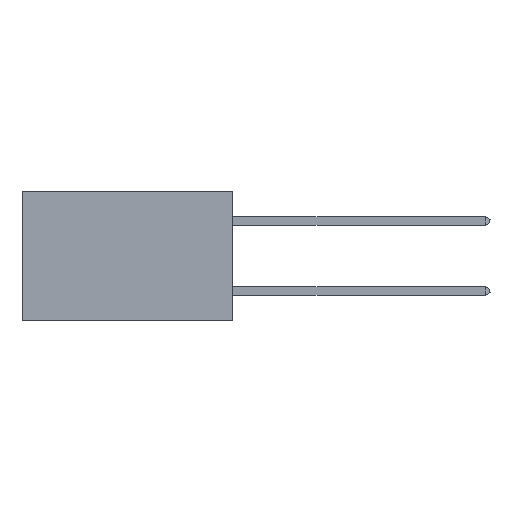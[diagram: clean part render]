
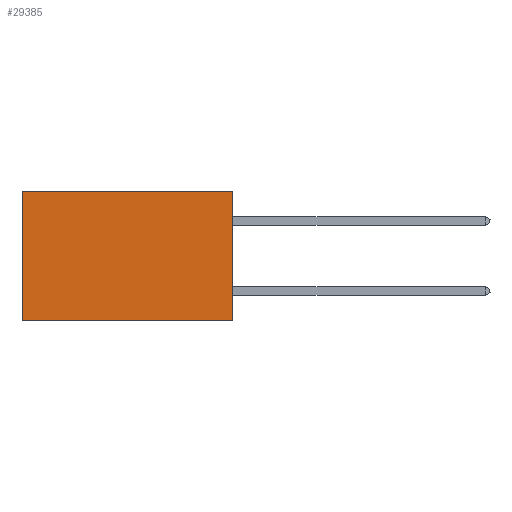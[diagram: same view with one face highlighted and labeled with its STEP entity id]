
A CAD part, left-side view. The second image highlights one B-rep face of the part: STEP entity #29385.
In plain terms, the highlighted planar face has unit normal (-1, 0, 0).
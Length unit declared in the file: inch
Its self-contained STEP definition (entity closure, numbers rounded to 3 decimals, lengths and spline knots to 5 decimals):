
#735 = VERTEX_POINT ( 'NONE', #17103 ) ;
#1496 = DIRECTION ( 'NONE',  ( 1., 0., 0. ) ) ;
#2989 = AXIS2_PLACEMENT_3D ( 'NONE', #29914, #1496, #18304 ) ;
#3746 = ORIENTED_EDGE ( 'NONE', *, *, #8281, .F. ) ;
#4450 = DIRECTION ( 'NONE',  ( 0., 0., -1. ) ) ;
#5558 = ORIENTED_EDGE ( 'NONE', *, *, #13737, .T. ) ;
#6247 = CARTESIAN_POINT ( 'NONE',  ( 0.2875, 0.6, -0.37 ) ) ;
#6467 = EDGE_LOOP ( 'NONE', ( #12537, #3746, #24023, #5558 ) ) ;
#7039 = VERTEX_POINT ( 'NONE', #28938 ) ;
#8281 = EDGE_CURVE ( 'NONE', #7039, #26730, #9430, .T. ) ;
#8569 = CARTESIAN_POINT ( 'NONE',  ( 0.2875, 0., 0. ) ) ;
#9321 = CARTESIAN_POINT ( 'NONE',  ( 0.2875, 0.6, 0. ) ) ;
#9430 = LINE ( 'NONE', #9608, #15730 ) ;
#9608 = CARTESIAN_POINT ( 'NONE',  ( 0.2875, 0., -0.37 ) ) ;
#11564 = LINE ( 'NONE', #14207, #23347 ) ;
#11989 = DIRECTION ( 'NONE',  ( 0., 1., 0. ) ) ;
#12326 = CARTESIAN_POINT ( 'NONE',  ( 0.2875, 0.6, 0. ) ) ;
#12537 = ORIENTED_EDGE ( 'NONE', *, *, #26924, .T. ) ;
#12671 = FACE_OUTER_BOUND ( 'NONE', #6467, .T. ) ;
#13186 = VECTOR ( 'NONE', #22706, 39.37008 ) ;
#13737 = EDGE_CURVE ( 'NONE', #735, #23566, #11564, .T. ) ;
#14207 = CARTESIAN_POINT ( 'NONE',  ( 0.2875, 0., 0. ) ) ;
#15730 = VECTOR ( 'NONE', #11989, 39.37008 ) ;
#16586 = DIRECTION ( 'NONE',  ( 0., 1., 0. ) ) ;
#17103 = CARTESIAN_POINT ( 'NONE',  ( 0.2875, 0., 0. ) ) ;
#17999 = LINE ( 'NONE', #8569, #13186 ) ;
#18304 = DIRECTION ( 'NONE',  ( 0., 0., -1. ) ) ;
#18772 = LINE ( 'NONE', #9321, #24263 ) ;
#22706 = DIRECTION ( 'NONE',  ( 0., 0., -1. ) ) ;
#23347 = VECTOR ( 'NONE', #16586, 39.37008 ) ;
#23566 = VERTEX_POINT ( 'NONE', #12326 ) ;
#24023 = ORIENTED_EDGE ( 'NONE', *, *, #27376, .F. ) ;
#24263 = VECTOR ( 'NONE', #4450, 39.37008 ) ;
#26730 = VERTEX_POINT ( 'NONE', #6247 ) ;
#26924 = EDGE_CURVE ( 'NONE', #23566, #26730, #18772, .T. ) ;
#27376 = EDGE_CURVE ( 'NONE', #735, #7039, #17999, .T. ) ;
#27568 = PLANE ( 'NONE',  #2989 ) ;
#28938 = CARTESIAN_POINT ( 'NONE',  ( 0.2875, 0., -0.37 ) ) ;
#29385 = ADVANCED_FACE ( 'NONE', ( #12671 ), #27568, .F. ) ;
#29914 = CARTESIAN_POINT ( 'NONE',  ( 0.2875, 0., 0. ) ) ;
